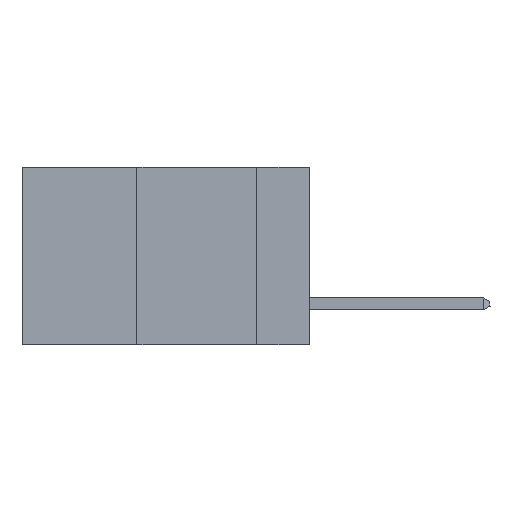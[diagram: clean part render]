
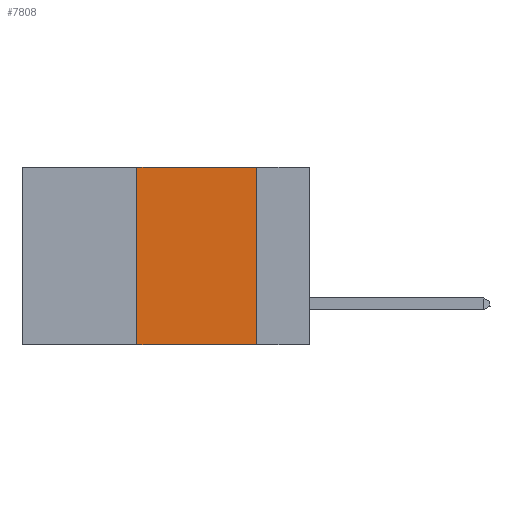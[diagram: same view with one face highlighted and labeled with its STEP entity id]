
A CAD part, left-side view. The second image highlights one B-rep face of the part: STEP entity #7808.
In plain terms, the highlighted planar face has unit normal (-1, 0, 0).
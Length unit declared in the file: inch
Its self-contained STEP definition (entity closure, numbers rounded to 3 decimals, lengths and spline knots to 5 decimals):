
#368 = VECTOR ( 'NONE', #12615, 39.37008 ) ;
#464 = VECTOR ( 'NONE', #10911, 39.37008 ) ;
#1312 = EDGE_LOOP ( 'NONE', ( #19014, #9240, #2045, #8058 ) ) ;
#1635 = CARTESIAN_POINT ( 'NONE',  ( 0., 0.6, 0. ) ) ;
#2045 = ORIENTED_EDGE ( 'NONE', *, *, #10729, .F. ) ;
#2536 = LINE ( 'NONE', #18003, #15895 ) ;
#3112 = VERTEX_POINT ( 'NONE', #15114 ) ;
#3486 = VERTEX_POINT ( 'NONE', #9839 ) ;
#3757 = EDGE_CURVE ( 'NONE', #4658, #3112, #6943, .T. ) ;
#3797 = LINE ( 'NONE', #14991, #11249 ) ;
#4606 = DIRECTION ( 'NONE',  ( 0., 0., -1. ) ) ;
#4658 = VERTEX_POINT ( 'NONE', #18923 ) ;
#4696 = LINE ( 'NONE', #10847, #464 ) ;
#6131 = PLANE ( 'NONE',  #10219 ) ;
#6262 = EDGE_CURVE ( 'NONE', #3486, #17764, #2536, .T. ) ;
#6377 = EDGE_CURVE ( 'NONE', #3112, #17764, #4696, .T. ) ;
#6943 = LINE ( 'NONE', #17088, #368 ) ;
#7808 = ADVANCED_FACE ( 'NONE', ( #19093 ), #6131, .F. ) ;
#8058 = ORIENTED_EDGE ( 'NONE', *, *, #6262, .T. ) ;
#9240 = ORIENTED_EDGE ( 'NONE', *, *, #3757, .F. ) ;
#9839 = CARTESIAN_POINT ( 'NONE',  ( 0., 0.36, -0.37 ) ) ;
#10219 = AXIS2_PLACEMENT_3D ( 'NONE', #1635, #16499, #4606 ) ;
#10409 = DIRECTION ( 'NONE',  ( 0., 0., 1. ) ) ;
#10587 = DIRECTION ( 'NONE',  ( 0., -1., 0. ) ) ;
#10729 = EDGE_CURVE ( 'NONE', #3486, #4658, #3797, .T. ) ;
#10847 = CARTESIAN_POINT ( 'NONE',  ( 0., 0.11, 0. ) ) ;
#10911 = DIRECTION ( 'NONE',  ( 0., 0., -1. ) ) ;
#11249 = VECTOR ( 'NONE', #10409, 39.37008 ) ;
#11372 = CARTESIAN_POINT ( 'NONE',  ( 0., 0.11, -0.37 ) ) ;
#12615 = DIRECTION ( 'NONE',  ( 0., -1., 0. ) ) ;
#14991 = CARTESIAN_POINT ( 'NONE',  ( 0., 0.36, 0. ) ) ;
#15114 = CARTESIAN_POINT ( 'NONE',  ( 0., 0.11, 0. ) ) ;
#15895 = VECTOR ( 'NONE', #10587, 39.37008 ) ;
#16499 = DIRECTION ( 'NONE',  ( 1., 0., 0. ) ) ;
#17088 = CARTESIAN_POINT ( 'NONE',  ( 0., 0.6, 0. ) ) ;
#17764 = VERTEX_POINT ( 'NONE', #11372 ) ;
#18003 = CARTESIAN_POINT ( 'NONE',  ( 0., 0.6, -0.37 ) ) ;
#18923 = CARTESIAN_POINT ( 'NONE',  ( 0., 0.36, 0. ) ) ;
#19014 = ORIENTED_EDGE ( 'NONE', *, *, #6377, .F. ) ;
#19093 = FACE_OUTER_BOUND ( 'NONE', #1312, .T. ) ;
